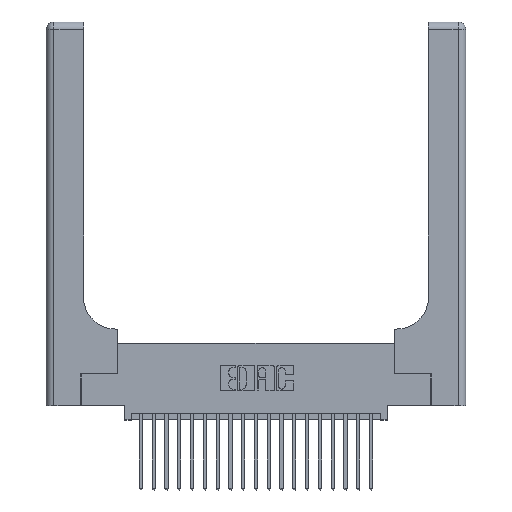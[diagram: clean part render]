
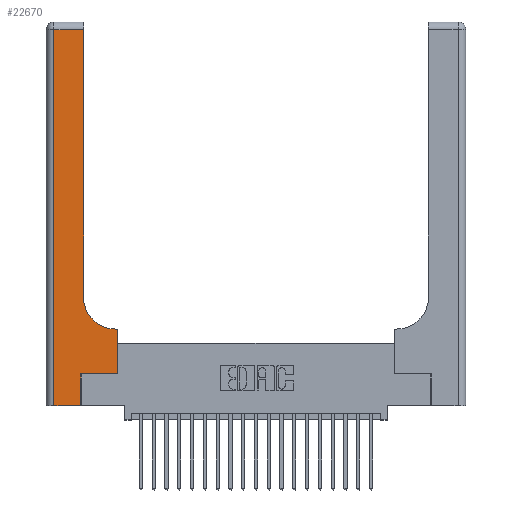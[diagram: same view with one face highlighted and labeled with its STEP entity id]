
A CAD part, top view. The second image highlights one B-rep face of the part: STEP entity #22670.
In plain terms, the highlighted planar face has unit normal (0, 0, 1).
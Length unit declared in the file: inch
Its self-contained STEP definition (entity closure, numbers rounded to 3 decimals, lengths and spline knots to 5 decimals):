
#119 = VERTEX_POINT ( 'NONE', #1694 ) ;
#314 = VECTOR ( 'NONE', #11951, 39.37008 ) ;
#442 = EDGE_CURVE ( 'NONE', #21725, #10674, #18902, .T. ) ;
#710 = CARTESIAN_POINT ( 'NONE',  ( 0.269, 0.25, 0.37 ) ) ;
#845 = ORIENTED_EDGE ( 'NONE', *, *, #10777, .T. ) ;
#982 = LINE ( 'NONE', #11454, #3236 ) ;
#1195 = CARTESIAN_POINT ( 'NONE',  ( 0.06, 2.94, 0.37 ) ) ;
#1274 = LINE ( 'NONE', #710, #18718 ) ;
#1281 = CARTESIAN_POINT ( 'NONE',  ( 0.5585, 0.6, 0.37 ) ) ;
#1293 = FACE_OUTER_BOUND ( 'NONE', #7404, .T. ) ;
#1409 = DIRECTION ( 'NONE',  ( -1., 0., 0. ) ) ;
#1437 = VERTEX_POINT ( 'NONE', #5454 ) ;
#1517 = DIRECTION ( 'NONE',  ( 0., 1., 0. ) ) ;
#1637 = CARTESIAN_POINT ( 'NONE',  ( 0.2915, 0.6, 0.37 ) ) ;
#1694 = CARTESIAN_POINT ( 'NONE',  ( 0.5415, 0.6, 0.37 ) ) ;
#1759 = CARTESIAN_POINT ( 'NONE',  ( 0.2915, 3., 0.37 ) ) ;
#2072 = LINE ( 'NONE', #22762, #3763 ) ;
#2393 = DIRECTION ( 'NONE',  ( 0., 1., 0. ) ) ;
#2967 = ORIENTED_EDGE ( 'NONE', *, *, #5747, .T. ) ;
#3226 = CARTESIAN_POINT ( 'NONE',  ( 0.06, 0., 0.37 ) ) ;
#3236 = VECTOR ( 'NONE', #2393, 39.37008 ) ;
#3346 = ORIENTED_EDGE ( 'NONE', *, *, #18568, .T. ) ;
#3406 = DIRECTION ( 'NONE',  ( 0., 0., -1. ) ) ;
#3490 = CARTESIAN_POINT ( 'NONE',  ( 0., 3., 0.37 ) ) ;
#3763 = VECTOR ( 'NONE', #1409, 39.37008 ) ;
#4717 = CIRCLE ( 'NONE', #20772, 0.25 ) ;
#5009 = EDGE_CURVE ( 'NONE', #22127, #7420, #982, .T. ) ;
#5454 = CARTESIAN_POINT ( 'NONE',  ( 0.2915, 2.94, 0.37 ) ) ;
#5555 = CARTESIAN_POINT ( 'NONE',  ( 0.5415, 0.85, 0.37 ) ) ;
#5747 = EDGE_CURVE ( 'NONE', #1437, #14370, #2072, .T. ) ;
#6119 = EDGE_CURVE ( 'NONE', #7886, #22127, #21712, .T. ) ;
#7404 = EDGE_LOOP ( 'NONE', ( #3346, #2967, #20106, #13009, #15388, #15582, #8388, #19023, #845 ) ) ;
#7420 = VERTEX_POINT ( 'NONE', #11940 ) ;
#7886 = VERTEX_POINT ( 'NONE', #3226 ) ;
#8388 = ORIENTED_EDGE ( 'NONE', *, *, #442, .T. ) ;
#8774 = CARTESIAN_POINT ( 'NONE',  ( 0.5585, 0.25, 0.37 ) ) ;
#8974 = EDGE_CURVE ( 'NONE', #14370, #7886, #17460, .T. ) ;
#9029 = DIRECTION ( 'NONE',  ( -1., 0., 0. ) ) ;
#9327 = VERTEX_POINT ( 'NONE', #14613 ) ;
#9364 = VECTOR ( 'NONE', #13169, 39.37008 ) ;
#10486 = VECTOR ( 'NONE', #1517, 39.37008 ) ;
#10674 = VERTEX_POINT ( 'NONE', #1281 ) ;
#10777 = EDGE_CURVE ( 'NONE', #119, #9327, #4717, .T. ) ;
#10917 = EDGE_CURVE ( 'NONE', #10674, #119, #10935, .T. ) ;
#10935 = LINE ( 'NONE', #1637, #11196 ) ;
#11020 = DIRECTION ( 'NONE',  ( -1., 0., 0. ) ) ;
#11196 = VECTOR ( 'NONE', #11020, 39.37008 ) ;
#11454 = CARTESIAN_POINT ( 'NONE',  ( 0.269, 0., 0.37 ) ) ;
#11940 = CARTESIAN_POINT ( 'NONE',  ( 0.269, 0.25, 0.37 ) ) ;
#11951 = DIRECTION ( 'NONE',  ( 0., -1., 0. ) ) ;
#13009 = ORIENTED_EDGE ( 'NONE', *, *, #6119, .T. ) ;
#13169 = DIRECTION ( 'NONE',  ( 0., 1., 0. ) ) ;
#13246 = DIRECTION ( 'NONE',  ( 1., 0., 0. ) ) ;
#14370 = VERTEX_POINT ( 'NONE', #1195 ) ;
#14613 = CARTESIAN_POINT ( 'NONE',  ( 0.2915, 0.85, 0.37 ) ) ;
#15388 = ORIENTED_EDGE ( 'NONE', *, *, #5009, .T. ) ;
#15582 = ORIENTED_EDGE ( 'NONE', *, *, #22964, .T. ) ;
#16150 = PLANE ( 'NONE',  #17379 ) ;
#16787 = CARTESIAN_POINT ( 'NONE',  ( 0.269, 0., 0.37 ) ) ;
#16955 = LINE ( 'NONE', #1759, #10486 ) ;
#17016 = CARTESIAN_POINT ( 'NONE',  ( 0.06, 3., 0.37 ) ) ;
#17224 = DIRECTION ( 'NONE',  ( 1., 0., 0. ) ) ;
#17379 = AXIS2_PLACEMENT_3D ( 'NONE', #3490, #3406, #9029 ) ;
#17460 = LINE ( 'NONE', #17016, #314 ) ;
#17749 = VECTOR ( 'NONE', #17224, 39.37008 ) ;
#18117 = DIRECTION ( 'NONE',  ( 0., 0., -1. ) ) ;
#18568 = EDGE_CURVE ( 'NONE', #9327, #1437, #16955, .T. ) ;
#18718 = VECTOR ( 'NONE', #13246, 39.37008 ) ;
#18902 = LINE ( 'NONE', #20092, #9364 ) ;
#19023 = ORIENTED_EDGE ( 'NONE', *, *, #10917, .T. ) ;
#19042 = CARTESIAN_POINT ( 'NONE',  ( 0., 0., 0.37 ) ) ;
#20016 = DIRECTION ( 'NONE',  ( 1., 0., 0. ) ) ;
#20092 = CARTESIAN_POINT ( 'NONE',  ( 0.5585, 0.25, 0.37 ) ) ;
#20106 = ORIENTED_EDGE ( 'NONE', *, *, #8974, .T. ) ;
#20772 = AXIS2_PLACEMENT_3D ( 'NONE', #5555, #18117, #20016 ) ;
#21712 = LINE ( 'NONE', #19042, #17749 ) ;
#21725 = VERTEX_POINT ( 'NONE', #8774 ) ;
#22127 = VERTEX_POINT ( 'NONE', #16787 ) ;
#22670 = ADVANCED_FACE ( 'NONE', ( #1293 ), #16150, .F. ) ;
#22762 = CARTESIAN_POINT ( 'NONE',  ( 0., 2.94, 0.37 ) ) ;
#22964 = EDGE_CURVE ( 'NONE', #7420, #21725, #1274, .T. ) ;
